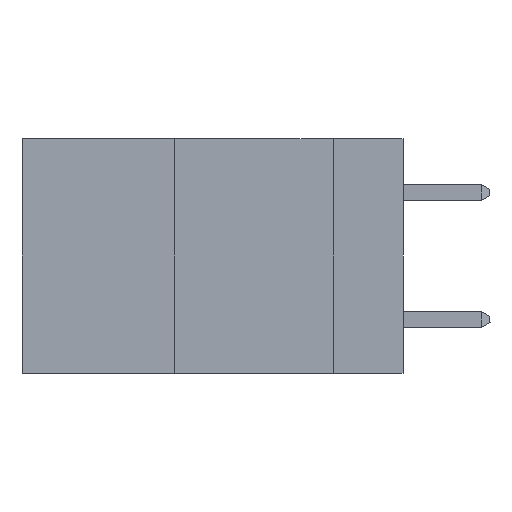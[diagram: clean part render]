
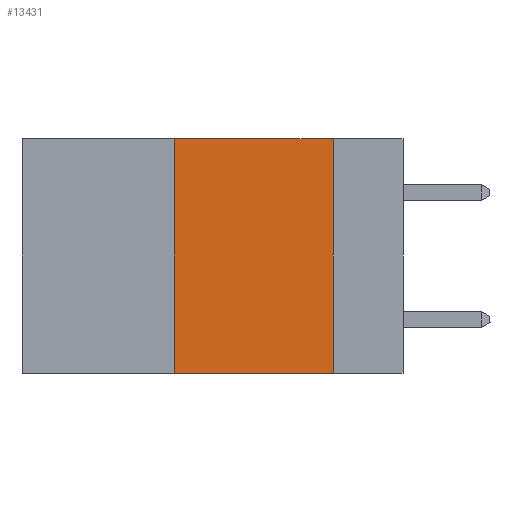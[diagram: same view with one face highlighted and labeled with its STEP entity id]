
A CAD part, left-side view. The second image highlights one B-rep face of the part: STEP entity #13431.
In plain terms, the highlighted planar face has unit normal (-1, 0, 0).
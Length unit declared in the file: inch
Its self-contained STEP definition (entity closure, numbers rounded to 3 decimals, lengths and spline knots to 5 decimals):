
#203 = EDGE_CURVE ( 'NONE', #748, #3454, #1436, .T. ) ;
#748 = VERTEX_POINT ( 'NONE', #8434 ) ;
#1436 = LINE ( 'NONE', #9791, #17836 ) ;
#1642 = EDGE_CURVE ( 'NONE', #23943, #3679, #26733, .T. ) ;
#2329 = CARTESIAN_POINT ( 'NONE',  ( 0., 0.36, 0. ) ) ;
#2667 = FACE_OUTER_BOUND ( 'NONE', #5762, .T. ) ;
#2810 = CARTESIAN_POINT ( 'NONE',  ( 0., 0.6, 0. ) ) ;
#3454 = VERTEX_POINT ( 'NONE', #13095 ) ;
#3521 = VECTOR ( 'NONE', #14277, 39.37008 ) ;
#3679 = VERTEX_POINT ( 'NONE', #25502 ) ;
#5762 = EDGE_LOOP ( 'NONE', ( #17331, #11155, #7740, #21720 ) ) ;
#7694 = CARTESIAN_POINT ( 'NONE',  ( 0., 0.36, 0. ) ) ;
#7740 = ORIENTED_EDGE ( 'NONE', *, *, #12742, .F. ) ;
#8434 = CARTESIAN_POINT ( 'NONE',  ( 0., 0.36, -0.37 ) ) ;
#8963 = DIRECTION ( 'NONE',  ( 1., 0., 0. ) ) ;
#9791 = CARTESIAN_POINT ( 'NONE',  ( 0., 0.6, -0.37 ) ) ;
#10999 = AXIS2_PLACEMENT_3D ( 'NONE', #2810, #8963, #25554 ) ;
#11135 = VECTOR ( 'NONE', #19709, 39.37008 ) ;
#11155 = ORIENTED_EDGE ( 'NONE', *, *, #1642, .F. ) ;
#11354 = CARTESIAN_POINT ( 'NONE',  ( 0., 0.11, 0. ) ) ;
#12742 = EDGE_CURVE ( 'NONE', #748, #23943, #21360, .T. ) ;
#12885 = DIRECTION ( 'NONE',  ( 0., 0., 1. ) ) ;
#13095 = CARTESIAN_POINT ( 'NONE',  ( 0., 0.11, -0.37 ) ) ;
#13431 = ADVANCED_FACE ( 'NONE', ( #2667 ), #15514, .F. ) ;
#13783 = DIRECTION ( 'NONE',  ( 0., -1., 0. ) ) ;
#14277 = DIRECTION ( 'NONE',  ( 0., -1., 0. ) ) ;
#15514 = PLANE ( 'NONE',  #10999 ) ;
#15563 = EDGE_CURVE ( 'NONE', #3679, #3454, #19312, .T. ) ;
#17331 = ORIENTED_EDGE ( 'NONE', *, *, #15563, .F. ) ;
#17836 = VECTOR ( 'NONE', #13783, 39.37008 ) ;
#19312 = LINE ( 'NONE', #11354, #11135 ) ;
#19709 = DIRECTION ( 'NONE',  ( 0., 0., -1. ) ) ;
#20135 = VECTOR ( 'NONE', #12885, 39.37008 ) ;
#21360 = LINE ( 'NONE', #2329, #20135 ) ;
#21720 = ORIENTED_EDGE ( 'NONE', *, *, #203, .T. ) ;
#23943 = VERTEX_POINT ( 'NONE', #7694 ) ;
#24693 = CARTESIAN_POINT ( 'NONE',  ( 0., 0.6, 0. ) ) ;
#25502 = CARTESIAN_POINT ( 'NONE',  ( 0., 0.11, 0. ) ) ;
#25554 = DIRECTION ( 'NONE',  ( 0., 0., -1. ) ) ;
#26733 = LINE ( 'NONE', #24693, #3521 ) ;
